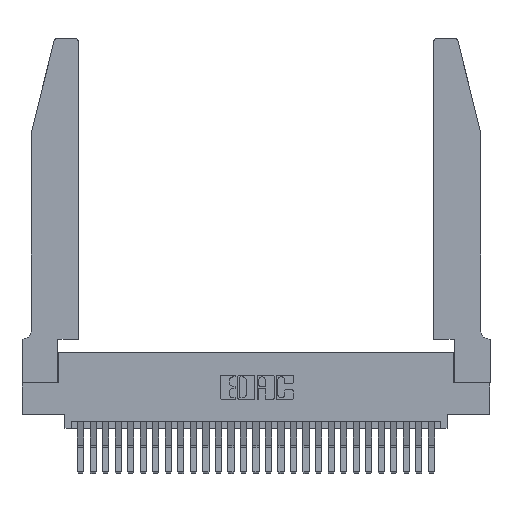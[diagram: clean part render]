
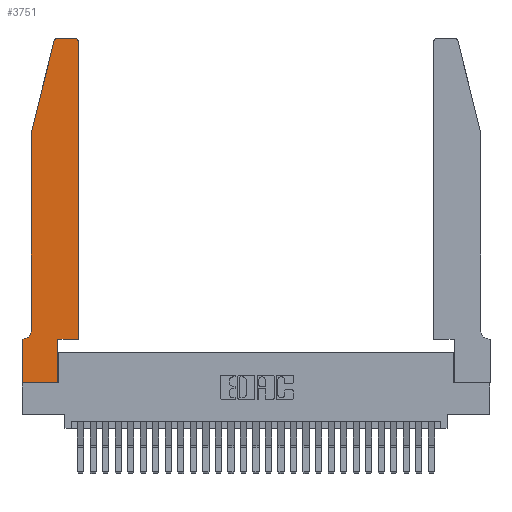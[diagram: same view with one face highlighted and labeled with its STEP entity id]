
A CAD part, top view. The second image highlights one B-rep face of the part: STEP entity #3751.
In plain terms, the highlighted planar face has unit normal (0, 0, 1).
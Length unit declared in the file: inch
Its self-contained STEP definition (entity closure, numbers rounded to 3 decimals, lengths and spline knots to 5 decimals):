
#630 = EDGE_CURVE ( 'NONE', #13319, #9539, #14882, .T. ) ;
#688 = EDGE_CURVE ( 'NONE', #10503, #22363, #13479, .T. ) ;
#950 = DIRECTION ( 'NONE',  ( 1., 0., 0. ) ) ;
#1493 = DIRECTION ( 'NONE',  ( 0., 0., 1. ) ) ;
#1646 = VECTOR ( 'NONE', #13865, 39.37008 ) ;
#1695 = LINE ( 'NONE', #27629, #3807 ) ;
#1846 = LINE ( 'NONE', #5162, #11111 ) ;
#2363 = CARTESIAN_POINT ( 'NONE',  ( 0.4505, 0.35, 0.37 ) ) ;
#2507 = ORIENTED_EDGE ( 'NONE', *, *, #16075, .T. ) ;
#2509 = VERTEX_POINT ( 'NONE', #25153 ) ;
#2590 = CARTESIAN_POINT ( 'NONE',  ( 0.2605, 2.75, 0.37 ) ) ;
#2696 = EDGE_CURVE ( 'NONE', #22363, #2509, #24441, .T. ) ;
#2944 = DIRECTION ( 'NONE',  ( 0., 0., 1. ) ) ;
#2950 = CARTESIAN_POINT ( 'NONE',  ( 0., 0., 0.37 ) ) ;
#3102 = DIRECTION ( 'NONE',  ( 1., 0., 0. ) ) ;
#3215 = CARTESIAN_POINT ( 'NONE',  ( 0.0755, 2., 0.37 ) ) ;
#3348 = DIRECTION ( 'NONE',  ( -1., 0., 0. ) ) ;
#3613 = ORIENTED_EDGE ( 'NONE', *, *, #20053, .T. ) ;
#3751 = ADVANCED_FACE ( 'NONE', ( #21129 ), #17475, .T. ) ;
#3807 = VECTOR ( 'NONE', #27078, 39.37008 ) ;
#4556 = CARTESIAN_POINT ( 'NONE',  ( 0.0755, 2., 0.37 ) ) ;
#4563 = DIRECTION ( 'NONE',  ( -1., 0., 0. ) ) ;
#4728 = CARTESIAN_POINT ( 'NONE',  ( 0., 0.35, 0.37 ) ) ;
#5080 = CARTESIAN_POINT ( 'NONE',  ( 0.4505, 0.35, 0.37 ) ) ;
#5162 = CARTESIAN_POINT ( 'NONE',  ( 0.0755, 2., 0.37 ) ) ;
#5809 = AXIS2_PLACEMENT_3D ( 'NONE', #19088, #7904, #23860 ) ;
#5884 = ORIENTED_EDGE ( 'NONE', *, *, #23063, .T. ) ;
#6531 = ORIENTED_EDGE ( 'NONE', *, *, #12891, .T. ) ;
#6682 = CARTESIAN_POINT ( 'NONE',  ( 0.2865, 0., 0.37 ) ) ;
#7154 = ORIENTED_EDGE ( 'NONE', *, *, #12617, .T. ) ;
#7443 = AXIS2_PLACEMENT_3D ( 'NONE', #24099, #1493, #24297 ) ;
#7810 = VERTEX_POINT ( 'NONE', #4728 ) ;
#7904 = DIRECTION ( 'NONE',  ( 0., 0., 1. ) ) ;
#9307 = VERTEX_POINT ( 'NONE', #24312 ) ;
#9520 = LINE ( 'NONE', #5080, #12017 ) ;
#9539 = VERTEX_POINT ( 'NONE', #6682 ) ;
#10385 = EDGE_CURVE ( 'NONE', #9307, #24961, #1846, .T. ) ;
#10392 = CIRCLE ( 'NONE', #7443, 0.03 ) ;
#10503 = VERTEX_POINT ( 'NONE', #25866 ) ;
#10564 = CARTESIAN_POINT ( 'NONE',  ( 0.2865, 0.35, 0.37 ) ) ;
#10910 = VERTEX_POINT ( 'NONE', #19819 ) ;
#11111 = VECTOR ( 'NONE', #14449, 39.37008 ) ;
#11567 = CARTESIAN_POINT ( 'NONE',  ( 0.0755, 0.35, 0.37 ) ) ;
#12017 = VECTOR ( 'NONE', #3102, 39.37008 ) ;
#12617 = EDGE_CURVE ( 'NONE', #21574, #10503, #1695, .T. ) ;
#12891 = EDGE_CURVE ( 'NONE', #25284, #21574, #9520, .T. ) ;
#13319 = VERTEX_POINT ( 'NONE', #19299 ) ;
#13333 = ORIENTED_EDGE ( 'NONE', *, *, #20292, .T. ) ;
#13458 = CARTESIAN_POINT ( 'NONE',  ( 0.0055, 0.35, 0.37 ) ) ;
#13479 = CIRCLE ( 'NONE', #5809, 0.03 ) ;
#13846 = VECTOR ( 'NONE', #950, 39.37008 ) ;
#13865 = DIRECTION ( 'NONE',  ( -1., 0., 0. ) ) ;
#14449 = DIRECTION ( 'NONE',  ( -0.239, -0.971, 0. ) ) ;
#14781 = DIRECTION ( 'NONE',  ( 0., -1., 0. ) ) ;
#14882 = LINE ( 'NONE', #2950, #13846 ) ;
#15019 = CARTESIAN_POINT ( 'NONE',  ( 0.2865, 0.35, 0.37 ) ) ;
#15143 = CARTESIAN_POINT ( 'NONE',  ( 0.4205, 2.75, 0.37 ) ) ;
#15211 = CIRCLE ( 'NONE', #19336, 0.07 ) ;
#15235 = LINE ( 'NONE', #11567, #29486 ) ;
#15716 = VECTOR ( 'NONE', #14781, 39.37008 ) ;
#16075 = EDGE_CURVE ( 'NONE', #18539, #7810, #15235, .T. ) ;
#16625 = LINE ( 'NONE', #10564, #18136 ) ;
#16650 = ORIENTED_EDGE ( 'NONE', *, *, #688, .T. ) ;
#17352 = LINE ( 'NONE', #25754, #18430 ) ;
#17475 = PLANE ( 'NONE',  #28354 ) ;
#17944 = ORIENTED_EDGE ( 'NONE', *, *, #23286, .T. ) ;
#18136 = VECTOR ( 'NONE', #19199, 39.37008 ) ;
#18430 = VECTOR ( 'NONE', #23379, 39.37008 ) ;
#18539 = VERTEX_POINT ( 'NONE', #13458 ) ;
#19088 = CARTESIAN_POINT ( 'NONE',  ( 0.4205, 2.72, 0.37 ) ) ;
#19199 = DIRECTION ( 'NONE',  ( 0., 1., 0. ) ) ;
#19299 = CARTESIAN_POINT ( 'NONE',  ( 0., 0., 0.37 ) ) ;
#19336 = AXIS2_PLACEMENT_3D ( 'NONE', #26469, #21971, #3348 ) ;
#19819 = CARTESIAN_POINT ( 'NONE',  ( 0.0755, 0.42, 0.37 ) ) ;
#20053 = EDGE_CURVE ( 'NONE', #9539, #25284, #16625, .T. ) ;
#20253 = ORIENTED_EDGE ( 'NONE', *, *, #20800, .T. ) ;
#20292 = EDGE_CURVE ( 'NONE', #2509, #9307, #10392, .T. ) ;
#20800 = EDGE_CURVE ( 'NONE', #24961, #10910, #23914, .T. ) ;
#21129 = FACE_OUTER_BOUND ( 'NONE', #24764, .T. ) ;
#21574 = VERTEX_POINT ( 'NONE', #2363 ) ;
#21971 = DIRECTION ( 'NONE',  ( 0., 0., -1. ) ) ;
#22363 = VERTEX_POINT ( 'NONE', #15143 ) ;
#22924 = ORIENTED_EDGE ( 'NONE', *, *, #10385, .T. ) ;
#23063 = EDGE_CURVE ( 'NONE', #7810, #13319, #17352, .T. ) ;
#23286 = EDGE_CURVE ( 'NONE', #10910, #18539, #15211, .T. ) ;
#23379 = DIRECTION ( 'NONE',  ( 0., -1., 0. ) ) ;
#23739 = ORIENTED_EDGE ( 'NONE', *, *, #630, .T. ) ;
#23860 = DIRECTION ( 'NONE',  ( 1., 0., 0. ) ) ;
#23914 = LINE ( 'NONE', #3215, #15716 ) ;
#23956 = DIRECTION ( 'NONE',  ( 1., 0., 0. ) ) ;
#24099 = CARTESIAN_POINT ( 'NONE',  ( 0.284, 2.72, 0.37 ) ) ;
#24297 = DIRECTION ( 'NONE',  ( 1., 0., 0. ) ) ;
#24312 = CARTESIAN_POINT ( 'NONE',  ( 0.25487, 2.72718, 0.37 ) ) ;
#24441 = LINE ( 'NONE', #2590, #1646 ) ;
#24764 = EDGE_LOOP ( 'NONE', ( #25852, #13333, #22924, #20253, #17944, #2507, #5884, #23739, #3613, #6531, #7154, #16650 ) ) ;
#24961 = VERTEX_POINT ( 'NONE', #4556 ) ;
#25153 = CARTESIAN_POINT ( 'NONE',  ( 0.284, 2.75, 0.37 ) ) ;
#25284 = VERTEX_POINT ( 'NONE', #15019 ) ;
#25754 = CARTESIAN_POINT ( 'NONE',  ( 0., 0., 0.37 ) ) ;
#25852 = ORIENTED_EDGE ( 'NONE', *, *, #2696, .T. ) ;
#25866 = CARTESIAN_POINT ( 'NONE',  ( 0.4505, 2.72, 0.37 ) ) ;
#26469 = CARTESIAN_POINT ( 'NONE',  ( 0.0055, 0.42, 0.37 ) ) ;
#27078 = DIRECTION ( 'NONE',  ( 0., 1., 0. ) ) ;
#27629 = CARTESIAN_POINT ( 'NONE',  ( 0.4505, 0.35, 0.37 ) ) ;
#27843 = CARTESIAN_POINT ( 'NONE',  ( 0., 0.35, 0.37 ) ) ;
#28354 = AXIS2_PLACEMENT_3D ( 'NONE', #27843, #2944, #23956 ) ;
#29486 = VECTOR ( 'NONE', #4563, 39.37008 ) ;
